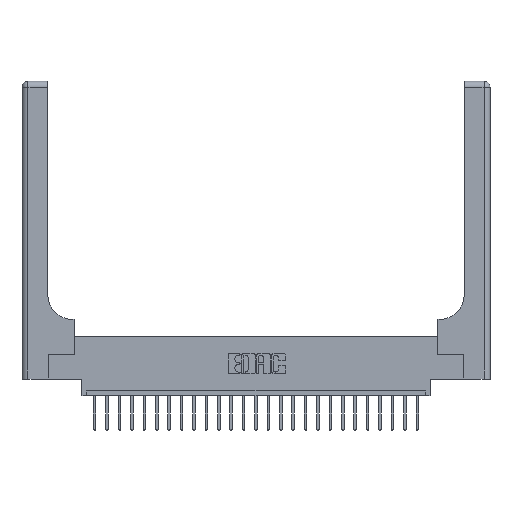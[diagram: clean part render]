
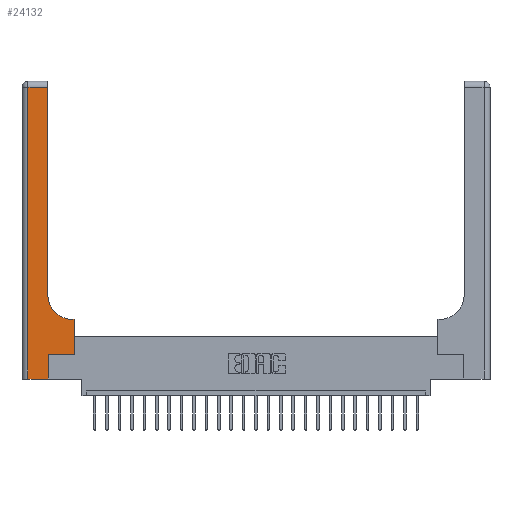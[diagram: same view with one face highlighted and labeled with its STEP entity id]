
A CAD part, top view. The second image highlights one B-rep face of the part: STEP entity #24132.
In plain terms, the highlighted planar face has unit normal (0, 0, 1).
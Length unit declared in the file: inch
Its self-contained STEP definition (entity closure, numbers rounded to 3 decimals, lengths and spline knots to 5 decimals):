
#35 = CARTESIAN_POINT ( 'NONE',  ( 0.51, 0.85, 0.37 ) ) ;
#828 = LINE ( 'NONE', #10027, #23194 ) ;
#1051 = CARTESIAN_POINT ( 'NONE',  ( 0.06, 0., 0.37 ) ) ;
#1239 = DIRECTION ( 'NONE',  ( -1., 0., 0. ) ) ;
#1324 = EDGE_LOOP ( 'NONE', ( #21176, #16614, #11573, #6183, #6182, #7409, #2463, #19406, #3441 ) ) ;
#1412 = EDGE_CURVE ( 'NONE', #3978, #6968, #6964, .T. ) ;
#1440 = CARTESIAN_POINT ( 'NONE',  ( 0., 3., 0.37 ) ) ;
#1565 = VECTOR ( 'NONE', #10590, 39.37008 ) ;
#1710 = CARTESIAN_POINT ( 'NONE',  ( 0.26, 2.94, 0.37 ) ) ;
#1720 = CARTESIAN_POINT ( 'NONE',  ( 0.26, 0.85, 0.37 ) ) ;
#2338 = AXIS2_PLACEMENT_3D ( 'NONE', #1440, #8775, #12987 ) ;
#2463 = ORIENTED_EDGE ( 'NONE', *, *, #7997, .T. ) ;
#2629 = CARTESIAN_POINT ( 'NONE',  ( 0.26, 0.6, 0.37 ) ) ;
#2910 = DIRECTION ( 'NONE',  ( 0., -1., 0. ) ) ;
#3332 = CARTESIAN_POINT ( 'NONE',  ( 0.265, 0., 0.37 ) ) ;
#3441 = ORIENTED_EDGE ( 'NONE', *, *, #5734, .T. ) ;
#3451 = LINE ( 'NONE', #22084, #14194 ) ;
#3493 = CARTESIAN_POINT ( 'NONE',  ( 0.51, 0.6, 0.37 ) ) ;
#3889 = VECTOR ( 'NONE', #1239, 39.37008 ) ;
#3978 = VERTEX_POINT ( 'NONE', #1710 ) ;
#4305 = DIRECTION ( 'NONE',  ( 0., 1., 0. ) ) ;
#4362 = CARTESIAN_POINT ( 'NONE',  ( 0., 0., 0.37 ) ) ;
#4739 = VERTEX_POINT ( 'NONE', #3493 ) ;
#4931 = PLANE ( 'NONE',  #2338 ) ;
#5316 = DIRECTION ( 'NONE',  ( 0., 1., 0. ) ) ;
#5734 = EDGE_CURVE ( 'NONE', #4739, #8532, #19222, .T. ) ;
#5799 = LINE ( 'NONE', #11522, #23591 ) ;
#6182 = ORIENTED_EDGE ( 'NONE', *, *, #18999, .T. ) ;
#6183 = ORIENTED_EDGE ( 'NONE', *, *, #9363, .T. ) ;
#6213 = VERTEX_POINT ( 'NONE', #13650 ) ;
#6345 = LINE ( 'NONE', #4362, #16788 ) ;
#6671 = EDGE_CURVE ( 'NONE', #6968, #23262, #10378, .T. ) ;
#6964 = LINE ( 'NONE', #8941, #3889 ) ;
#6968 = VERTEX_POINT ( 'NONE', #21378 ) ;
#7409 = ORIENTED_EDGE ( 'NONE', *, *, #18954, .T. ) ;
#7849 = DIRECTION ( 'NONE',  ( 0., 0., -1. ) ) ;
#7997 = EDGE_CURVE ( 'NONE', #6213, #11460, #16286, .T. ) ;
#8154 = CARTESIAN_POINT ( 'NONE',  ( 0.528, 0.6, 0.37 ) ) ;
#8532 = VERTEX_POINT ( 'NONE', #1720 ) ;
#8775 = DIRECTION ( 'NONE',  ( 0., 0., -1. ) ) ;
#8941 = CARTESIAN_POINT ( 'NONE',  ( 0., 2.94, 0.37 ) ) ;
#9363 = EDGE_CURVE ( 'NONE', #23262, #21434, #6345, .T. ) ;
#10027 = CARTESIAN_POINT ( 'NONE',  ( 0.265, 0., 0.37 ) ) ;
#10378 = LINE ( 'NONE', #16068, #18129 ) ;
#10590 = DIRECTION ( 'NONE',  ( 0., 1., 0. ) ) ;
#11246 = EDGE_CURVE ( 'NONE', #11460, #4739, #24204, .T. ) ;
#11460 = VERTEX_POINT ( 'NONE', #8154 ) ;
#11522 = CARTESIAN_POINT ( 'NONE',  ( 0.265, 0.25, 0.37 ) ) ;
#11573 = ORIENTED_EDGE ( 'NONE', *, *, #6671, .T. ) ;
#12186 = DIRECTION ( 'NONE',  ( 1., 0., 0. ) ) ;
#12987 = DIRECTION ( 'NONE',  ( -1., 0., 0. ) ) ;
#13497 = DIRECTION ( 'NONE',  ( 1., 0., 0. ) ) ;
#13650 = CARTESIAN_POINT ( 'NONE',  ( 0.528, 0.25, 0.37 ) ) ;
#14194 = VECTOR ( 'NONE', #5316, 39.37008 ) ;
#15692 = VECTOR ( 'NONE', #20349, 39.37008 ) ;
#16068 = CARTESIAN_POINT ( 'NONE',  ( 0.06, 3., 0.37 ) ) ;
#16286 = LINE ( 'NONE', #19770, #1565 ) ;
#16614 = ORIENTED_EDGE ( 'NONE', *, *, #1412, .T. ) ;
#16788 = VECTOR ( 'NONE', #12186, 39.37008 ) ;
#18046 = AXIS2_PLACEMENT_3D ( 'NONE', #35, #7849, #21253 ) ;
#18129 = VECTOR ( 'NONE', #2910, 39.37008 ) ;
#18570 = FACE_OUTER_BOUND ( 'NONE', #1324, .T. ) ;
#18954 = EDGE_CURVE ( 'NONE', #22512, #6213, #5799, .T. ) ;
#18999 = EDGE_CURVE ( 'NONE', #21434, #22512, #828, .T. ) ;
#19222 = CIRCLE ( 'NONE', #18046, 0.25 ) ;
#19406 = ORIENTED_EDGE ( 'NONE', *, *, #11246, .T. ) ;
#19770 = CARTESIAN_POINT ( 'NONE',  ( 0.528, 0.25, 0.37 ) ) ;
#20349 = DIRECTION ( 'NONE',  ( -1., 0., 0. ) ) ;
#20468 = CARTESIAN_POINT ( 'NONE',  ( 0.265, 0.25, 0.37 ) ) ;
#21176 = ORIENTED_EDGE ( 'NONE', *, *, #22504, .T. ) ;
#21253 = DIRECTION ( 'NONE',  ( 1., 0., 0. ) ) ;
#21378 = CARTESIAN_POINT ( 'NONE',  ( 0.06, 2.94, 0.37 ) ) ;
#21434 = VERTEX_POINT ( 'NONE', #3332 ) ;
#22084 = CARTESIAN_POINT ( 'NONE',  ( 0.26, 3., 0.37 ) ) ;
#22504 = EDGE_CURVE ( 'NONE', #8532, #3978, #3451, .T. ) ;
#22512 = VERTEX_POINT ( 'NONE', #20468 ) ;
#23194 = VECTOR ( 'NONE', #4305, 39.37008 ) ;
#23262 = VERTEX_POINT ( 'NONE', #1051 ) ;
#23591 = VECTOR ( 'NONE', #13497, 39.37008 ) ;
#24132 = ADVANCED_FACE ( 'NONE', ( #18570 ), #4931, .F. ) ;
#24204 = LINE ( 'NONE', #2629, #15692 ) ;
